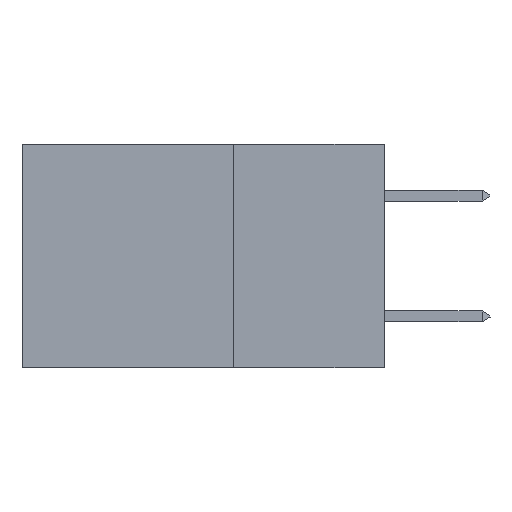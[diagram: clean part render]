
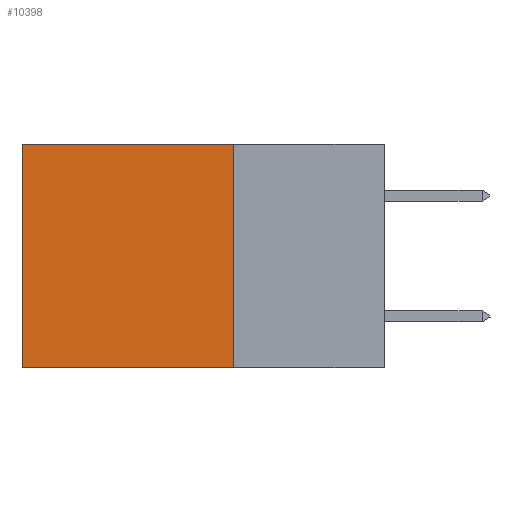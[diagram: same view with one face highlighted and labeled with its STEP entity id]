
A CAD part, left-side view. The second image highlights one B-rep face of the part: STEP entity #10398.
In plain terms, the highlighted planar face has unit normal (-1, 0, 0).
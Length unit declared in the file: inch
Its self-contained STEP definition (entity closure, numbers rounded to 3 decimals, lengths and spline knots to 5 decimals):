
#566 = CARTESIAN_POINT ( 'NONE',  ( 0.2875, 0.25, 0. ) ) ;
#715 = DIRECTION ( 'NONE',  ( 0., 0., -1. ) ) ;
#1139 = CARTESIAN_POINT ( 'NONE',  ( 0.2875, 0.25, 0. ) ) ;
#1355 = VERTEX_POINT ( 'NONE', #20479 ) ;
#2773 = CARTESIAN_POINT ( 'NONE',  ( 0.2875, 0.25, -0.37 ) ) ;
#3085 = DIRECTION ( 'NONE',  ( 0., 1., 0. ) ) ;
#3215 = VECTOR ( 'NONE', #715, 39.37008 ) ;
#6666 = DIRECTION ( 'NONE',  ( 0., 0., -1. ) ) ;
#7570 = VERTEX_POINT ( 'NONE', #12078 ) ;
#9317 = LINE ( 'NONE', #15250, #11248 ) ;
#9320 = VERTEX_POINT ( 'NONE', #2773 ) ;
#9351 = CARTESIAN_POINT ( 'NONE',  ( 0.2875, 0.25, 0. ) ) ;
#10398 = ADVANCED_FACE ( 'NONE', ( #22146 ), #19893, .F. ) ;
#11248 = VECTOR ( 'NONE', #3085, 39.37008 ) ;
#11931 = ORIENTED_EDGE ( 'NONE', *, *, #15052, .T. ) ;
#12025 = ORIENTED_EDGE ( 'NONE', *, *, #18970, .T. ) ;
#12078 = CARTESIAN_POINT ( 'NONE',  ( 0.2875, 0.6, -0.37 ) ) ;
#12701 = VECTOR ( 'NONE', #15050, 39.37008 ) ;
#12896 = EDGE_LOOP ( 'NONE', ( #12025, #17256, #16235, #11931 ) ) ;
#13885 = LINE ( 'NONE', #18659, #17999 ) ;
#14313 = EDGE_CURVE ( 'NONE', #9320, #7570, #16534, .T. ) ;
#14611 = DIRECTION ( 'NONE',  ( 1., 0., 0. ) ) ;
#15050 = DIRECTION ( 'NONE',  ( 0., 1., 0. ) ) ;
#15052 = EDGE_CURVE ( 'NONE', #21138, #1355, #9317, .T. ) ;
#15250 = CARTESIAN_POINT ( 'NONE',  ( 0.2875, 0.25, 0. ) ) ;
#16235 = ORIENTED_EDGE ( 'NONE', *, *, #16634, .F. ) ;
#16534 = LINE ( 'NONE', #18569, #12701 ) ;
#16634 = EDGE_CURVE ( 'NONE', #21138, #9320, #21623, .T. ) ;
#17256 = ORIENTED_EDGE ( 'NONE', *, *, #14313, .F. ) ;
#17999 = VECTOR ( 'NONE', #6666, 39.37008 ) ;
#18295 = DIRECTION ( 'NONE',  ( 0., 0., -1. ) ) ;
#18569 = CARTESIAN_POINT ( 'NONE',  ( 0.2875, 0.25, -0.37 ) ) ;
#18659 = CARTESIAN_POINT ( 'NONE',  ( 0.2875, 0.6, 0. ) ) ;
#18970 = EDGE_CURVE ( 'NONE', #1355, #7570, #13885, .T. ) ;
#19893 = PLANE ( 'NONE',  #20757 ) ;
#20479 = CARTESIAN_POINT ( 'NONE',  ( 0.2875, 0.6, 0. ) ) ;
#20757 = AXIS2_PLACEMENT_3D ( 'NONE', #9351, #14611, #18295 ) ;
#21138 = VERTEX_POINT ( 'NONE', #1139 ) ;
#21623 = LINE ( 'NONE', #566, #3215 ) ;
#22146 = FACE_OUTER_BOUND ( 'NONE', #12896, .T. ) ;
